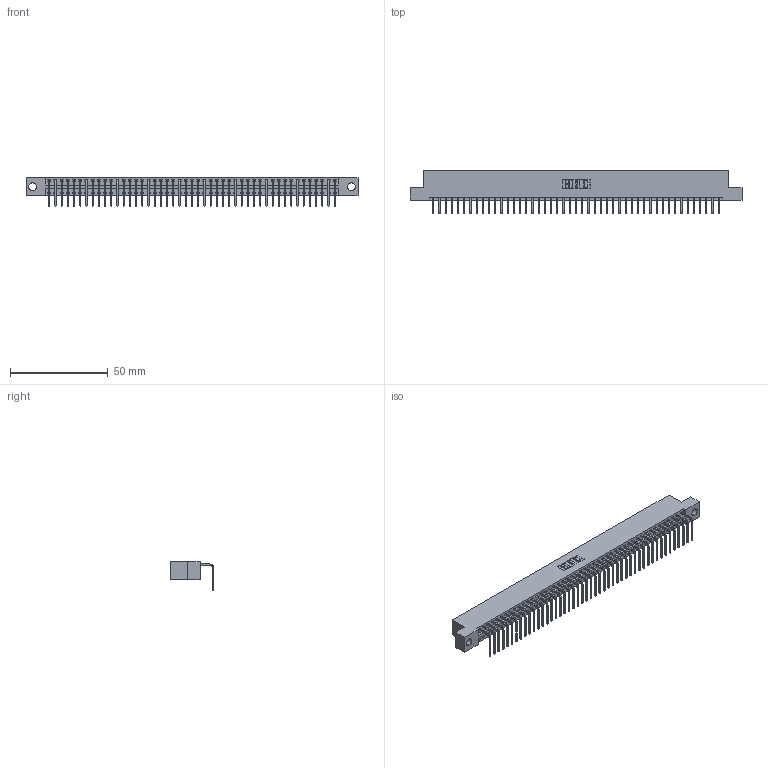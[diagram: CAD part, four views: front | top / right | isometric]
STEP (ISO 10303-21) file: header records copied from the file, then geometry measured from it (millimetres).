
FILE_DESCRIPTION (( 'STEP AP203' ), '1' );
FILE_NAME ('346-047-558-104.STEP', '2022-05-09T22:18:57', ( '' ), ( '' ), 'SwSTEP 2.0', 'SolidWorks 2020', '' );
FILE_SCHEMA (( 'CONFIG_CONTROL_DESIGN' ));
Length unit declared in the file: inch
Products named in the file (3): 346 Part_Flush Mounting Lugs - 0.156 Dia-TH; 345-292-001_558 Tail - 2; 346-047-558-104
Assembly tree (48 placements, depth 2):
  346-047-558-104
    346 Part_Flush Mounting Lugs - 0.156 Dia-TH
    345-292-001_558 Tail - 2  x47
Bounding box: 169.8 x 22.16 x 14.73 mm (x, y, z)
Volume: 16338.6 mm3; surface area: 21246.6 mm2
Topology: 48 solids, 48 shells, 2956 faces, 8919 edges, 5882 vertices
Faces by surface type: plane 2064, cylinder 892
Entity records: 28999 total; most frequent: CARTESIAN_POINT 4979, ORIENTED_EDGE 4958, DIRECTION 4385, EDGE_CURVE 2479, LINE 2159, VECTOR 2159, VERTEX_POINT 1650, AXIS2_PLACEMENT_3D 1113
